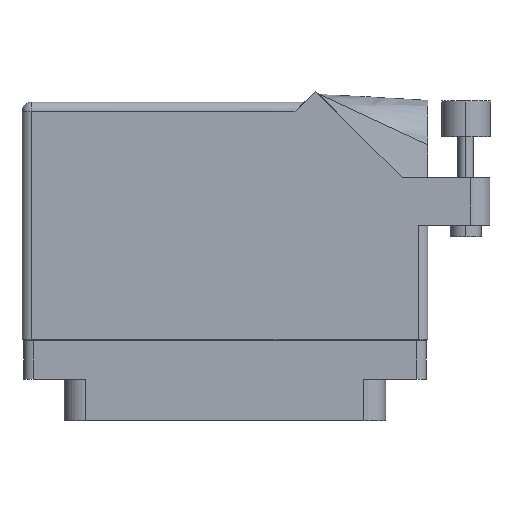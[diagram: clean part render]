
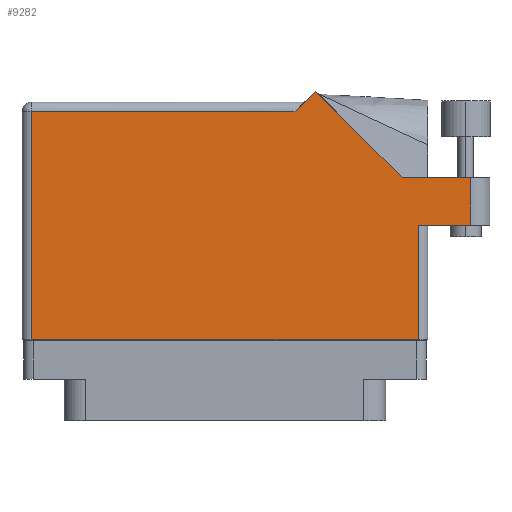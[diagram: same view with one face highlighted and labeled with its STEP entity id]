
A CAD part, front view. The second image highlights one B-rep face of the part: STEP entity #9282.
In plain terms, the highlighted face is planar.
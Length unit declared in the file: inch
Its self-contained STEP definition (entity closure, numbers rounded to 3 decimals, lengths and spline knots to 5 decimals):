
#1101 = VERTEX_POINT ( 'NONE', #22916 ) ;
#1559 = DIRECTION ( 'NONE',  ( 0., 0., -1. ) ) ;
#1731 = VERTEX_POINT ( 'NONE', #4874 ) ;
#2377 = DIRECTION ( 'NONE',  ( 0., 1., 0. ) ) ;
#2561 = VERTEX_POINT ( 'NONE', #13700 ) ;
#2848 = ORIENTED_EDGE ( 'NONE', *, *, #23452, .T. ) ;
#3375 = CARTESIAN_POINT ( 'NONE',  ( 1.581, 0.944, 0.455 ) ) ;
#3641 = EDGE_CURVE ( 'NONE', #42868, #13754, #18474, .T. ) ;
#4874 = CARTESIAN_POINT ( 'NONE',  ( 1.244, 0.637, 0.455 ) ) ;
#5012 = LINE ( 'NONE', #26640, #27609 ) ;
#5603 = CARTESIAN_POINT ( 'NONE',  ( -1.306, -0.1, 0.455 ) ) ;
#5773 = CARTESIAN_POINT ( 'NONE',  ( 1.14042, 0.944, 0.455 ) ) ;
#6810 = DIRECTION ( 'NONE',  ( -1., 0., 0. ) ) ;
#7212 = ORIENTED_EDGE ( 'NONE', *, *, #14217, .T. ) ;
#7301 = ORIENTED_EDGE ( 'NONE', *, *, #48612, .T. ) ;
#9282 = ADVANCED_FACE ( 'NONE', ( #38355 ), #49546, .F. ) ;
#9451 = EDGE_CURVE ( 'NONE', #49445, #42868, #5012, .T. ) ;
#10193 = AXIS2_PLACEMENT_3D ( 'NONE', #25636, #1559, #49385 ) ;
#10409 = LINE ( 'NONE', #39730, #41788 ) ;
#11840 = LINE ( 'NONE', #13883, #51900 ) ;
#13700 = CARTESIAN_POINT ( 'NONE',  ( -1.244, 1.368, 0.455 ) ) ;
#13754 = VERTEX_POINT ( 'NONE', #31311 ) ;
#13883 = CARTESIAN_POINT ( 'NONE',  ( -1.306, 1.368, 0.455 ) ) ;
#14217 = EDGE_CURVE ( 'NONE', #2561, #39863, #44777, .T. ) ;
#14352 = ORIENTED_EDGE ( 'NONE', *, *, #20185, .T. ) ;
#15638 = LINE ( 'NONE', #5603, #46333 ) ;
#15933 = ORIENTED_EDGE ( 'NONE', *, *, #47731, .T. ) ;
#16916 = EDGE_LOOP ( 'NONE', ( #7301, #42627, #43920, #37784, #15933, #14352, #7212, #33471, #2848 ) ) ;
#16987 = DIRECTION ( 'NONE',  ( -0.707, 0.707, 0. ) ) ;
#17306 = DIRECTION ( 'NONE',  ( 0., -1., 0. ) ) ;
#17522 = EDGE_CURVE ( 'NONE', #39863, #23409, #15638, .T. ) ;
#18203 = DIRECTION ( 'NONE',  ( -1., 0., 0. ) ) ;
#18362 = VECTOR ( 'NONE', #26193, 39.37008 ) ;
#18474 = LINE ( 'NONE', #20898, #39273 ) ;
#20185 = EDGE_CURVE ( 'NONE', #1101, #2561, #11840, .T. ) ;
#20898 = CARTESIAN_POINT ( 'NONE',  ( 1.14042, 0.944, 0.455 ) ) ;
#21684 = VECTOR ( 'NONE', #17306, 39.37008 ) ;
#22398 = CARTESIAN_POINT ( 'NONE',  ( -1.244, -0.1, 0.455 ) ) ;
#22916 = CARTESIAN_POINT ( 'NONE',  ( 0.451, 1.368, 0.455 ) ) ;
#23409 = VERTEX_POINT ( 'NONE', #26445 ) ;
#23452 = EDGE_CURVE ( 'NONE', #23409, #1731, #37174, .T. ) ;
#24115 = DIRECTION ( 'NONE',  ( -0.707, -0.707, 0. ) ) ;
#24487 = LINE ( 'NONE', #3375, #32629 ) ;
#25636 = CARTESIAN_POINT ( 'NONE',  ( -1.306, 1.43, 0.455 ) ) ;
#26193 = DIRECTION ( 'NONE',  ( 1., 0., 0. ) ) ;
#26445 = CARTESIAN_POINT ( 'NONE',  ( 1.244, -0.1, 0.455 ) ) ;
#26640 = CARTESIAN_POINT ( 'NONE',  ( 1.706, 0.944, 0.455 ) ) ;
#27609 = VECTOR ( 'NONE', #6810, 39.37008 ) ;
#31160 = DIRECTION ( 'NONE',  ( 0., 1., 0. ) ) ;
#31311 = CARTESIAN_POINT ( 'NONE',  ( 0.58371, 1.50071, 0.455 ) ) ;
#32629 = VECTOR ( 'NONE', #31160, 39.37008 ) ;
#33471 = ORIENTED_EDGE ( 'NONE', *, *, #17522, .T. ) ;
#35009 = CARTESIAN_POINT ( 'NONE',  ( 1.244, 0.637, 0.455 ) ) ;
#37174 = LINE ( 'NONE', #35009, #43985 ) ;
#37784 = ORIENTED_EDGE ( 'NONE', *, *, #3641, .T. ) ;
#38355 = FACE_OUTER_BOUND ( 'NONE', #16916, .T. ) ;
#39273 = VECTOR ( 'NONE', #16987, 39.37008 ) ;
#39730 = CARTESIAN_POINT ( 'NONE',  ( 0.513, 1.43, 0.455 ) ) ;
#39863 = VERTEX_POINT ( 'NONE', #22398 ) ;
#40970 = CARTESIAN_POINT ( 'NONE',  ( 1.581, 0.637, 0.455 ) ) ;
#41047 = CARTESIAN_POINT ( 'NONE',  ( -1.244, -0.1, 0.455 ) ) ;
#41788 = VECTOR ( 'NONE', #24115, 39.37008 ) ;
#42417 = VERTEX_POINT ( 'NONE', #40970 ) ;
#42627 = ORIENTED_EDGE ( 'NONE', *, *, #50879, .T. ) ;
#42868 = VERTEX_POINT ( 'NONE', #5773 ) ;
#43920 = ORIENTED_EDGE ( 'NONE', *, *, #9451, .T. ) ;
#43985 = VECTOR ( 'NONE', #2377, 39.37008 ) ;
#44178 = CARTESIAN_POINT ( 'NONE',  ( 1.581, 0.944, 0.455 ) ) ;
#44777 = LINE ( 'NONE', #41047, #21684 ) ;
#45846 = DIRECTION ( 'NONE',  ( 1., 0., 0. ) ) ;
#46333 = VECTOR ( 'NONE', #45846, 39.37008 ) ;
#47731 = EDGE_CURVE ( 'NONE', #13754, #1101, #10409, .T. ) ;
#47823 = LINE ( 'NONE', #49945, #18362 ) ;
#48612 = EDGE_CURVE ( 'NONE', #1731, #42417, #47823, .T. ) ;
#49385 = DIRECTION ( 'NONE',  ( -1., 0., 0. ) ) ;
#49445 = VERTEX_POINT ( 'NONE', #44178 ) ;
#49546 = PLANE ( 'NONE',  #10193 ) ;
#49945 = CARTESIAN_POINT ( 'NONE',  ( 1.306, 0.637, 0.455 ) ) ;
#50879 = EDGE_CURVE ( 'NONE', #42417, #49445, #24487, .T. ) ;
#51900 = VECTOR ( 'NONE', #18203, 39.37008 ) ;
